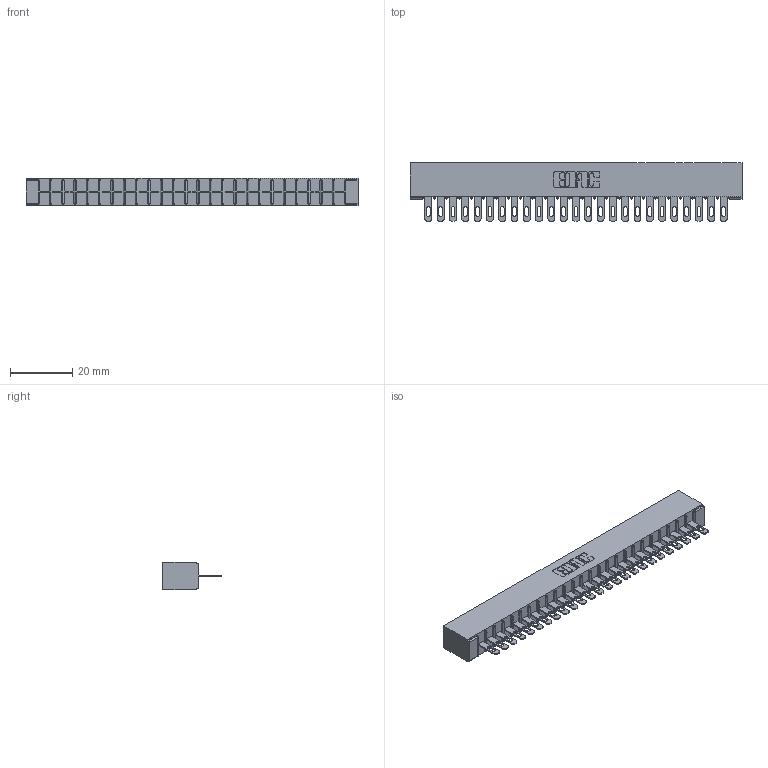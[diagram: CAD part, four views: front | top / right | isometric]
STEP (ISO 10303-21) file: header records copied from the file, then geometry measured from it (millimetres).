
FILE_DESCRIPTION (( 'STEP AP203' ), '1' );
FILE_NAME ('306-025-400-101.STEP', '2020-09-21T22:30:21', ( '' ), ( '' ), 'SwSTEP 2.0', 'SolidWorks 2020', '' );
FILE_SCHEMA (( 'CONFIG_CONTROL_DESIGN' ));
Length unit declared in the file: inch
Products named in the file (3): 306 Part_No Mounting; 306-290-001_100; 306-025-400-101
Assembly tree (26 placements, depth 2):
  306-025-400-101
    306 Part_No Mounting
    306-290-001_100  x25
Bounding box: 106.93 x 18.87 x 8.71 mm (x, y, z)
Volume: 7679.7 mm3; surface area: 12114.7 mm2
Topology: 26 solids, 26 shells, 2008 faces, 5667 edges, 3642 vertices
Faces by surface type: plane 1314, cylinder 594, sphere 100
Entity records: 25402 total; most frequent: CARTESIAN_POINT 4262, ORIENTED_EDGE 4222, DIRECTION 4205, EDGE_CURVE 2111, VECTOR 1643, LINE 1643, VERTEX_POINT 1338, AXIS2_PLACEMENT_3D 1281
